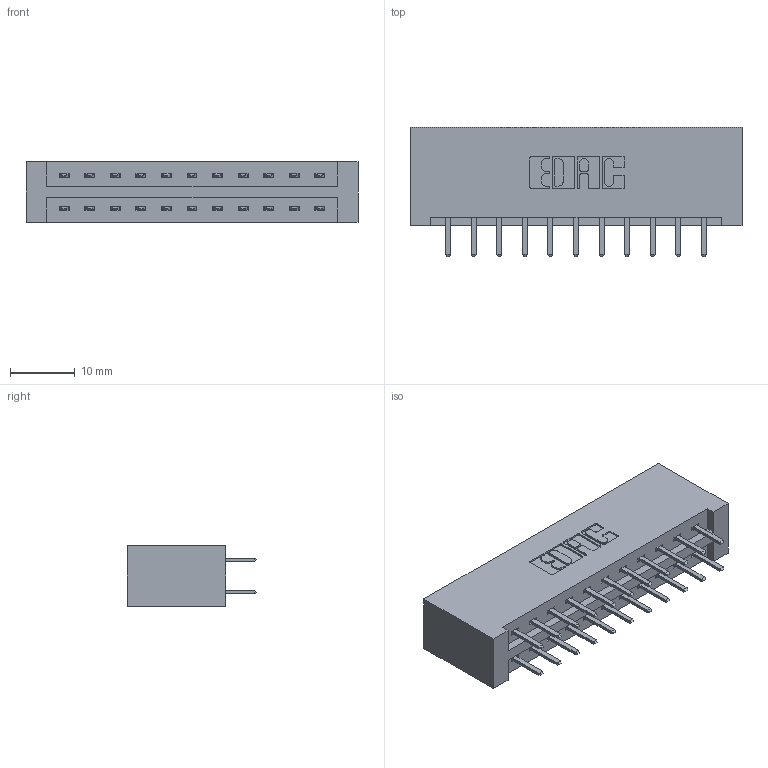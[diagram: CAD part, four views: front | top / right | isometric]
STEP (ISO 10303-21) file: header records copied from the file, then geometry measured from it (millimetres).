
FILE_DESCRIPTION (( 'STEP AP203' ), '1' );
FILE_NAME ('387-022-520-201.STEP', '2019-10-16T16:13:45', ( '' ), ( '' ), 'SwSTEP 2.0', 'SolidWorks 2016', '' );
FILE_SCHEMA (( 'CONFIG_CONTROL_DESIGN' ));
Length unit declared in the file: inch
Products named in the file (3): 345-292-001_345-293-120; 387-022-520-201; 337 Part_No Mounting Lugs
Assembly tree (23 placements, depth 2):
  387-022-520-201
    337 Part_No Mounting Lugs
    345-292-001_345-293-120  x22
Bounding box: 51.46 x 20.02 x 9.4 mm (x, y, z)
Volume: 5761.7 mm3; surface area: 6241 mm2
Topology: 23 solids, 23 shells, 1382 faces, 4005 edges, 2610 vertices
Faces by surface type: plane 946, cylinder 436
Entity records: 12375 total; most frequent: CARTESIAN_POINT 2122, ORIENTED_EDGE 2046, DIRECTION 1843, EDGE_CURVE 1023, LINE 899, VECTOR 899, VERTEX_POINT 678, AXIS2_PLACEMENT_3D 472
